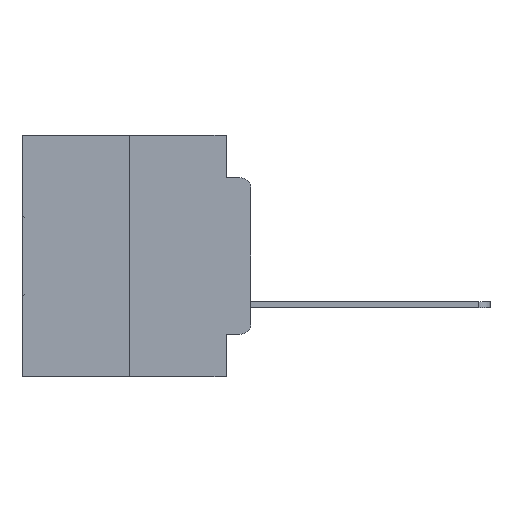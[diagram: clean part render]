
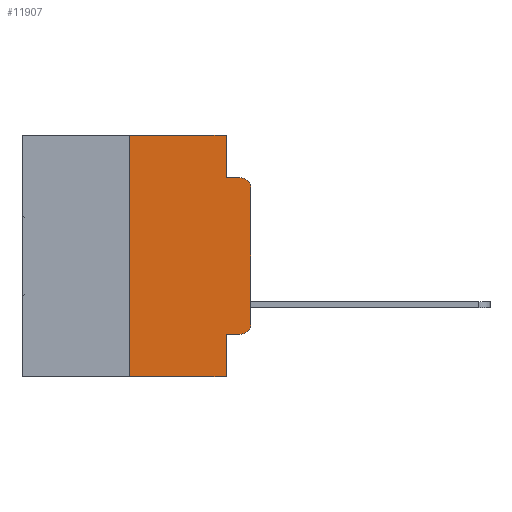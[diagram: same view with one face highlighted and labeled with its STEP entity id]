
A CAD part, left-side view. The second image highlights one B-rep face of the part: STEP entity #11907.
In plain terms, the highlighted planar face has unit normal (-1, 0, 0).
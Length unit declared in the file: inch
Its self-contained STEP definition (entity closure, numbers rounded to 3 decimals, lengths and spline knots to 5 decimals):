
#364 = CARTESIAN_POINT ( 'NONE',  ( 0., 0.051, -0.0885 ) ) ;
#556 = LINE ( 'NONE', #364, #30518 ) ;
#879 = CARTESIAN_POINT ( 'NONE',  ( 0., 0.25, -0.5 ) ) ;
#913 = CARTESIAN_POINT ( 'NONE',  ( 0., 0.051, -0.5 ) ) ;
#935 = DIRECTION ( 'NONE',  ( 0., 0., -1. ) ) ;
#1053 = VERTEX_POINT ( 'NONE', #22872 ) ;
#1206 = ORIENTED_EDGE ( 'NONE', *, *, #29151, .T. ) ;
#1302 = EDGE_CURVE ( 'NONE', #24996, #17748, #16643, .T. ) ;
#1308 = VERTEX_POINT ( 'NONE', #879 ) ;
#1812 = CARTESIAN_POINT ( 'NONE',  ( 0., 0., -0.3915 ) ) ;
#2413 = ORIENTED_EDGE ( 'NONE', *, *, #11818, .F. ) ;
#3176 = AXIS2_PLACEMENT_3D ( 'NONE', #3262, #21043, #5807 ) ;
#3262 = CARTESIAN_POINT ( 'NONE',  ( 0., 0.473, 0. ) ) ;
#3420 = CARTESIAN_POINT ( 'NONE',  ( 0., 0.473, -0.5 ) ) ;
#3705 = ORIENTED_EDGE ( 'NONE', *, *, #1302, .F. ) ;
#4593 = CARTESIAN_POINT ( 'NONE',  ( 0., 0., -0.1085 ) ) ;
#4879 = LINE ( 'NONE', #27390, #11017 ) ;
#5235 = PLANE ( 'NONE',  #3176 ) ;
#5259 = VERTEX_POINT ( 'NONE', #4593 ) ;
#5807 = DIRECTION ( 'NONE',  ( 0., 0., -1. ) ) ;
#5952 = DIRECTION ( 'NONE',  ( 0., -1., 0. ) ) ;
#6307 = ORIENTED_EDGE ( 'NONE', *, *, #16581, .T. ) ;
#7065 = CARTESIAN_POINT ( 'NONE',  ( 0., 0., 0. ) ) ;
#7386 = VECTOR ( 'NONE', #22933, 39.37008 ) ;
#10813 = DIRECTION ( 'NONE',  ( 0., -1., 0. ) ) ;
#10892 = DIRECTION ( 'NONE',  ( -1., 0., 0. ) ) ;
#11017 = VECTOR ( 'NONE', #32061, 39.37008 ) ;
#11598 = VERTEX_POINT ( 'NONE', #14236 ) ;
#11818 = EDGE_CURVE ( 'NONE', #11598, #22764, #4879, .T. ) ;
#11893 = CARTESIAN_POINT ( 'NONE',  ( 0., 0.02, -0.0885 ) ) ;
#11907 = ADVANCED_FACE ( 'NONE', ( #19092 ), #5235, .F. ) ;
#12145 = CIRCLE ( 'NONE', #27247, 0.02 ) ;
#12429 = CARTESIAN_POINT ( 'NONE',  ( 0., 0.051, -0.0885 ) ) ;
#12491 = ORIENTED_EDGE ( 'NONE', *, *, #23891, .T. ) ;
#12547 = CARTESIAN_POINT ( 'NONE',  ( 0., 0.02, -0.3915 ) ) ;
#12579 = VERTEX_POINT ( 'NONE', #1812 ) ;
#12854 = VECTOR ( 'NONE', #19048, 39.37008 ) ;
#13647 = LINE ( 'NONE', #16530, #12854 ) ;
#13836 = EDGE_CURVE ( 'NONE', #23453, #21927, #556, .T. ) ;
#14236 = CARTESIAN_POINT ( 'NONE',  ( 0., 0.25, 0. ) ) ;
#14877 = EDGE_CURVE ( 'NONE', #22764, #23453, #21527, .T. ) ;
#15139 = DIRECTION ( 'NONE',  ( 0., 0., -1. ) ) ;
#15421 = LINE ( 'NONE', #7065, #20472 ) ;
#15745 = EDGE_CURVE ( 'NONE', #12579, #5259, #15421, .T. ) ;
#15813 = ORIENTED_EDGE ( 'NONE', *, *, #15745, .T. ) ;
#16047 = DIRECTION ( 'NONE',  ( 0., 0., -1. ) ) ;
#16263 = LINE ( 'NONE', #3420, #21998 ) ;
#16530 = CARTESIAN_POINT ( 'NONE',  ( 0., 0.051, -0.4115 ) ) ;
#16581 = EDGE_CURVE ( 'NONE', #5259, #21927, #12145, .T. ) ;
#16643 = LINE ( 'NONE', #24981, #29463 ) ;
#17322 = ORIENTED_EDGE ( 'NONE', *, *, #14877, .F. ) ;
#17748 = VERTEX_POINT ( 'NONE', #913 ) ;
#17859 = CIRCLE ( 'NONE', #31720, 0.02 ) ;
#18080 = ORIENTED_EDGE ( 'NONE', *, *, #29594, .T. ) ;
#19048 = DIRECTION ( 'NONE',  ( 0., -1., 0. ) ) ;
#19092 = FACE_OUTER_BOUND ( 'NONE', #26279, .T. ) ;
#19650 = CARTESIAN_POINT ( 'NONE',  ( 0., 0.051, 0. ) ) ;
#20069 = VECTOR ( 'NONE', #935, 39.37008 ) ;
#20472 = VECTOR ( 'NONE', #24681, 39.37008 ) ;
#21043 = DIRECTION ( 'NONE',  ( 1., 0., 0. ) ) ;
#21527 = LINE ( 'NONE', #25973, #20069 ) ;
#21645 = LINE ( 'NONE', #30123, #7386 ) ;
#21927 = VERTEX_POINT ( 'NONE', #11893 ) ;
#21998 = VECTOR ( 'NONE', #5952, 39.37008 ) ;
#22010 = CARTESIAN_POINT ( 'NONE',  ( 0., 0.051, -0.4115 ) ) ;
#22764 = VERTEX_POINT ( 'NONE', #19650 ) ;
#22872 = CARTESIAN_POINT ( 'NONE',  ( 0., 0.02, -0.4115 ) ) ;
#22933 = DIRECTION ( 'NONE',  ( 0., 0., 1. ) ) ;
#23453 = VERTEX_POINT ( 'NONE', #12429 ) ;
#23891 = EDGE_CURVE ( 'NONE', #24996, #1053, #13647, .T. ) ;
#24681 = DIRECTION ( 'NONE',  ( 0., 0., 1. ) ) ;
#24981 = CARTESIAN_POINT ( 'NONE',  ( 0., 0.051, 0. ) ) ;
#24996 = VERTEX_POINT ( 'NONE', #22010 ) ;
#25721 = CARTESIAN_POINT ( 'NONE',  ( 0., 0.02, -0.1085 ) ) ;
#25973 = CARTESIAN_POINT ( 'NONE',  ( 0., 0.051, 0. ) ) ;
#26279 = EDGE_LOOP ( 'NONE', ( #15813, #6307, #29338, #17322, #2413, #30807, #1206, #3705, #12491, #18080 ) ) ;
#26542 = EDGE_CURVE ( 'NONE', #1308, #11598, #21645, .T. ) ;
#27247 = AXIS2_PLACEMENT_3D ( 'NONE', #25721, #10892, #28138 ) ;
#27390 = CARTESIAN_POINT ( 'NONE',  ( 0., 0.473, 0. ) ) ;
#28138 = DIRECTION ( 'NONE',  ( 0., 0., -1. ) ) ;
#29151 = EDGE_CURVE ( 'NONE', #1308, #17748, #16263, .T. ) ;
#29338 = ORIENTED_EDGE ( 'NONE', *, *, #13836, .F. ) ;
#29463 = VECTOR ( 'NONE', #16047, 39.37008 ) ;
#29594 = EDGE_CURVE ( 'NONE', #1053, #12579, #17859, .T. ) ;
#29649 = DIRECTION ( 'NONE',  ( -1., 0., 0. ) ) ;
#30123 = CARTESIAN_POINT ( 'NONE',  ( 0., 0.25, 0. ) ) ;
#30518 = VECTOR ( 'NONE', #10813, 39.37008 ) ;
#30807 = ORIENTED_EDGE ( 'NONE', *, *, #26542, .F. ) ;
#31720 = AXIS2_PLACEMENT_3D ( 'NONE', #12547, #29649, #15139 ) ;
#32061 = DIRECTION ( 'NONE',  ( 0., -1., 0. ) ) ;
